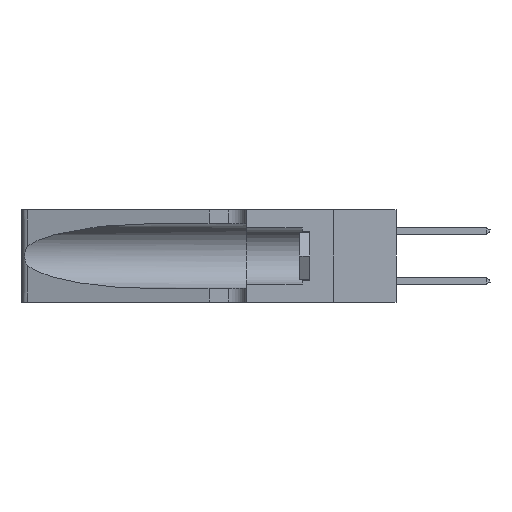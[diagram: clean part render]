
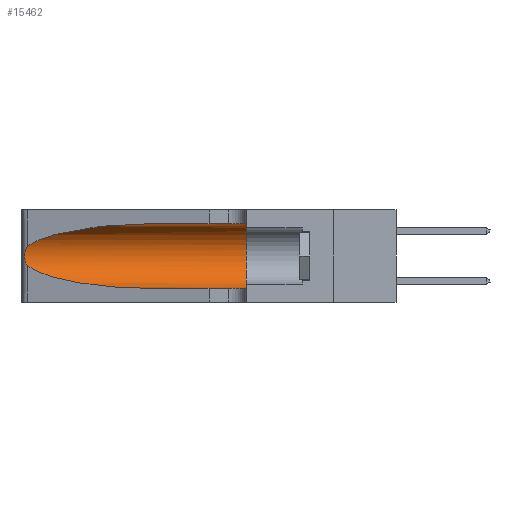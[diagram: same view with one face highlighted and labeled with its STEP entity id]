
A CAD part, left-side view. The second image highlights one B-rep face of the part: STEP entity #15462.
In plain terms, the highlighted cylindrical face has radius 3.308 mm (diameter 6.617 mm), a partial arc.
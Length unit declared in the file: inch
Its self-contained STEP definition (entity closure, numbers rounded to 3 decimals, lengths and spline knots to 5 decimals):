
#141 = CARTESIAN_POINT ( 'NONE',  ( 0.1305, 0.35, 0.31525 ) ) ;
#946 = CARTESIAN_POINT ( 'NONE',  ( 0.1305, 1.61858, 0.185 ) ) ;
#1410 = CARTESIAN_POINT ( 'NONE',  ( 0.1305, 1.61858, 0.05475 ) ) ;
#1428 = EDGE_CURVE ( 'NONE', #13400, #12413, #16661, .T. ) ;
#1921 = VECTOR ( 'NONE', #2576, 39.37008 ) ;
#2381 = CARTESIAN_POINT ( 'NONE',  ( 0.25856, 1.23593, 0.16098 ) ) ;
#2576 = DIRECTION ( 'NONE',  ( 0., -1., 0. ) ) ;
#3348 = B_SPLINE_CURVE_WITH_KNOTS ( 'NONE', 3,
 ( #4007, #10880, #7550, #12718, #10798, #21382, #19589, #11024, #17766, #2381, #4158, #12491, #5697, #21306 ),
 .UNSPECIFIED., .F., .F.,
 ( 4, 2, 2, 2, 2, 2, 4 ),
 ( 0., 0.00027, 0.00053, 0.00107, 0.0016, 0.00187, 0.00214 ),
 .UNSPECIFIED. ) ;
#3773 = EDGE_CURVE ( 'NONE', #12413, #10825, #4572, .T. ) ;
#3809 = EDGE_CURVE ( 'NONE', #13272, #10825, #11765, .T. ) ;
#3964 = EDGE_CURVE ( 'NONE', #13798, #13272, #8826, .T. ) ;
#4007 = CARTESIAN_POINT ( 'NONE',  ( 0.25487, 1.22718, 0.22369 ) ) ;
#4158 = CARTESIAN_POINT ( 'NONE',  ( 0.25789, 1.23486, 0.15765 ) ) ;
#4357 = CARTESIAN_POINT ( 'NONE',  ( 0.1305, 1.61858, 0.31525 ) ) ;
#4549 = CARTESIAN_POINT ( 'NONE',  ( 0.1305, 0.72297, 0.31525 ) ) ;
#4572 = LINE ( 'NONE', #1410, #12285 ) ;
#4924 = FACE_OUTER_BOUND ( 'NONE', #21227, .T. ) ;
#5152 = CARTESIAN_POINT ( 'NONE',  ( 0.1305, 0.72297, 0.31525 ) ) ;
#5697 = CARTESIAN_POINT ( 'NONE',  ( 0.25555, 1.22993, 0.14849 ) ) ;
#6258 = ORIENTED_EDGE ( 'NONE', *, *, #3773, .T. ) ;
#7213 = ORIENTED_EDGE ( 'NONE', *, *, #1428, .T. ) ;
#7550 = CARTESIAN_POINT ( 'NONE',  ( 0.25639, 1.23184, 0.21858 ) ) ;
#7733 = DIRECTION ( 'NONE',  ( 0., 0., -1. ) ) ;
#7956 = CARTESIAN_POINT ( 'NONE',  ( 0.2373, 1.15595, 0.28018 ) ) ;
#8515 = CARTESIAN_POINT ( 'NONE',  ( 0.1305, 0.35, 0.185 ) ) ;
#8826 = LINE ( 'NONE', #4357, #1921 ) ;
#9558 = ORIENTED_EDGE ( 'NONE', *, *, #19110, .T. ) ;
#10312 = DIRECTION ( 'NONE',  ( 0., 0., 1. ) ) ;
#10704 = VERTEX_POINT ( 'NONE', #20362 ) ;
#10798 = CARTESIAN_POINT ( 'NONE',  ( 0.25854, 1.2359, 0.20912 ) ) ;
#10825 = VERTEX_POINT ( 'NONE', #12784 ) ;
#10880 = CARTESIAN_POINT ( 'NONE',  ( 0.25555, 1.22994, 0.2215 ) ) ;
#11024 = CARTESIAN_POINT ( 'NONE',  ( 0.26075, 1.23896, 0.178 ) ) ;
#11765 = CIRCLE ( 'NONE', #17833, 0.13025 ) ;
#12285 = VECTOR ( 'NONE', #20244, 39.37008 ) ;
#12413 = VERTEX_POINT ( 'NONE', #16759 ) ;
#12491 = CARTESIAN_POINT ( 'NONE',  ( 0.25639, 1.23186, 0.15144 ) ) ;
#12718 = CARTESIAN_POINT ( 'NONE',  ( 0.25787, 1.23484, 0.2124 ) ) ;
#12751 = CARTESIAN_POINT ( 'NONE',  ( 0.2373, 1.15595, 0.08982 ) ) ;
#12784 = CARTESIAN_POINT ( 'NONE',  ( 0.1305, 0.35, 0.05475 ) ) ;
#12834 = DIRECTION ( 'NONE',  ( 0., -1., 0. ) ) ;
#13165 = ORIENTED_EDGE ( 'NONE', *, *, #3964, .F. ) ;
#13272 = VERTEX_POINT ( 'NONE', #141 ) ;
#13400 = VERTEX_POINT ( 'NONE', #19336 ) ;
#13798 = VERTEX_POINT ( 'NONE', #5152 ) ;
#13891 =( BOUNDED_CURVE ( )  B_SPLINE_CURVE ( 3, ( #4549, #16546, #7956, #18023 ),
 .UNSPECIFIED., .F., .F. ) 
 B_SPLINE_CURVE_WITH_KNOTS ( ( 4, 4 ),
 ( 1.5708, 2.84003 ),
 .UNSPECIFIED. ) 
 CURVE ( )  GEOMETRIC_REPRESENTATION_ITEM ( )  RATIONAL_B_SPLINE_CURVE ( ( 1., 0.87, 0.87, 1. ) ) 
 REPRESENTATION_ITEM ( '' )  );
#14428 = CARTESIAN_POINT ( 'NONE',  ( 0.25487, 1.22718, 0.14631 ) ) ;
#14587 = CYLINDRICAL_SURFACE ( 'NONE', #19632, 0.13025 ) ;
#14858 = ORIENTED_EDGE ( 'NONE', *, *, #16270, .T. ) ;
#15462 = ADVANCED_FACE ( 'NONE', ( #4924 ), #14587, .F. ) ;
#16270 = EDGE_CURVE ( 'NONE', #13798, #10704, #13891, .T. ) ;
#16389 = CARTESIAN_POINT ( 'NONE',  ( 0.1305, 0.72297, 0.05475 ) ) ;
#16546 = CARTESIAN_POINT ( 'NONE',  ( 0.18966, 0.96281, 0.31525 ) ) ;
#16661 =( BOUNDED_CURVE ( )  B_SPLINE_CURVE ( 3, ( #14428, #12751, #19765, #16389 ),
 .UNSPECIFIED., .F., .F. ) 
 B_SPLINE_CURVE_WITH_KNOTS ( ( 4, 4 ),
 ( 3.44316, 4.71239 ),
 .UNSPECIFIED. ) 
 CURVE ( )  GEOMETRIC_REPRESENTATION_ITEM ( )  RATIONAL_B_SPLINE_CURVE ( ( 1., 0.87, 0.87, 1. ) ) 
 REPRESENTATION_ITEM ( '' )  );
#16759 = CARTESIAN_POINT ( 'NONE',  ( 0.1305, 0.72297, 0.05475 ) ) ;
#17766 = CARTESIAN_POINT ( 'NONE',  ( 0.26017, 1.23833, 0.17102 ) ) ;
#17833 = AXIS2_PLACEMENT_3D ( 'NONE', #8515, #20529, #10312 ) ;
#18023 = CARTESIAN_POINT ( 'NONE',  ( 0.25487, 1.22718, 0.22369 ) ) ;
#19110 = EDGE_CURVE ( 'NONE', #10704, #13400, #3348, .T. ) ;
#19336 = CARTESIAN_POINT ( 'NONE',  ( 0.25487, 1.22718, 0.14631 ) ) ;
#19572 = ORIENTED_EDGE ( 'NONE', *, *, #3809, .F. ) ;
#19589 = CARTESIAN_POINT ( 'NONE',  ( 0.26075, 1.23896, 0.19203 ) ) ;
#19632 = AXIS2_PLACEMENT_3D ( 'NONE', #946, #12834, #7733 ) ;
#19765 = CARTESIAN_POINT ( 'NONE',  ( 0.18966, 0.96281, 0.05475 ) ) ;
#20244 = DIRECTION ( 'NONE',  ( 0., -1., 0. ) ) ;
#20362 = CARTESIAN_POINT ( 'NONE',  ( 0.25487, 1.22718, 0.22369 ) ) ;
#20529 = DIRECTION ( 'NONE',  ( 0., 1., 0. ) ) ;
#21227 = EDGE_LOOP ( 'NONE', ( #14858, #9558, #7213, #6258, #19572, #13165 ) ) ;
#21306 = CARTESIAN_POINT ( 'NONE',  ( 0.25487, 1.22718, 0.14631 ) ) ;
#21382 = CARTESIAN_POINT ( 'NONE',  ( 0.26018, 1.23835, 0.19895 ) ) ;
